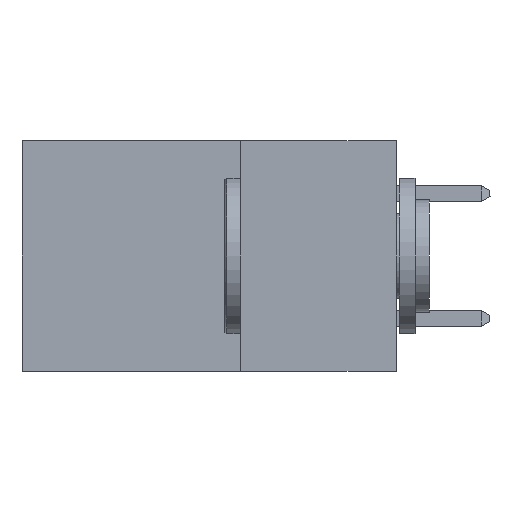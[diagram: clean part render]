
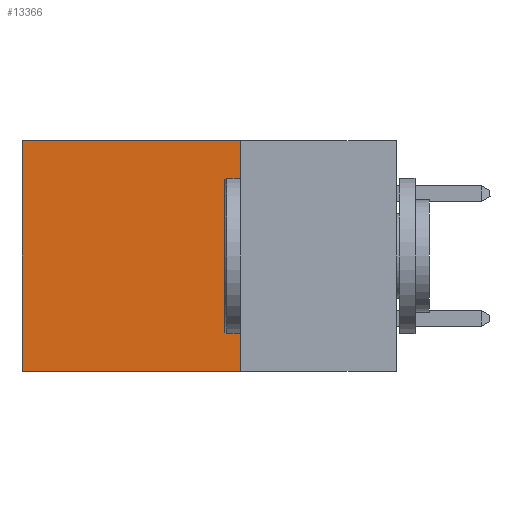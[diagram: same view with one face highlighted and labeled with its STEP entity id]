
A CAD part, left-side view. The second image highlights one B-rep face of the part: STEP entity #13366.
In plain terms, the highlighted planar face has unit normal (-1, 0, 0).
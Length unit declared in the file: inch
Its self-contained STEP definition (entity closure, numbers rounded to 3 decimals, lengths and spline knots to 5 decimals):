
#892 = CARTESIAN_POINT ( 'NONE',  ( 0.298, 0.6, 0. ) ) ;
#2331 = EDGE_CURVE ( 'NONE', #17434, #15738, #8246, .T. ) ;
#3453 = EDGE_CURVE ( 'NONE', #25049, #17434, #6326, .T. ) ;
#4589 = PLANE ( 'NONE',  #15478 ) ;
#4840 = VECTOR ( 'NONE', #21084, 39.37008 ) ;
#6326 = LINE ( 'NONE', #29854, #23415 ) ;
#7138 = DIRECTION ( 'NONE',  ( 0., 1., 0. ) ) ;
#7396 = CARTESIAN_POINT ( 'NONE',  ( 0.298, 0.25, -0.37 ) ) ;
#8246 = LINE ( 'NONE', #11074, #10422 ) ;
#9672 = ORIENTED_EDGE ( 'NONE', *, *, #22484, .T. ) ;
#10234 = ORIENTED_EDGE ( 'NONE', *, *, #16487, .T. ) ;
#10422 = VECTOR ( 'NONE', #7138, 39.37008 ) ;
#11074 = CARTESIAN_POINT ( 'NONE',  ( 0.298, 0.25, -0.37 ) ) ;
#11639 = DIRECTION ( 'NONE',  ( 1., 0., 0. ) ) ;
#12233 = VECTOR ( 'NONE', #15366, 39.37008 ) ;
#12458 = CARTESIAN_POINT ( 'NONE',  ( 0.298, 0.25, 0. ) ) ;
#13366 = ADVANCED_FACE ( 'NONE', ( #21396 ), #4589, .F. ) ;
#13510 = ORIENTED_EDGE ( 'NONE', *, *, #2331, .F. ) ;
#14886 = ORIENTED_EDGE ( 'NONE', *, *, #3453, .F. ) ;
#15366 = DIRECTION ( 'NONE',  ( 0., 0., -1. ) ) ;
#15471 = DIRECTION ( 'NONE',  ( 0., 0., -1. ) ) ;
#15478 = AXIS2_PLACEMENT_3D ( 'NONE', #20868, #11639, #27815 ) ;
#15738 = VERTEX_POINT ( 'NONE', #19323 ) ;
#16260 = EDGE_LOOP ( 'NONE', ( #10234, #13510, #14886, #9672 ) ) ;
#16487 = EDGE_CURVE ( 'NONE', #18747, #15738, #24560, .T. ) ;
#17434 = VERTEX_POINT ( 'NONE', #7396 ) ;
#18747 = VERTEX_POINT ( 'NONE', #892 ) ;
#19323 = CARTESIAN_POINT ( 'NONE',  ( 0.298, 0.6, -0.37 ) ) ;
#20868 = CARTESIAN_POINT ( 'NONE',  ( 0.298, 0.25, 0. ) ) ;
#21084 = DIRECTION ( 'NONE',  ( 0., 1., 0. ) ) ;
#21396 = FACE_OUTER_BOUND ( 'NONE', #16260, .T. ) ;
#22484 = EDGE_CURVE ( 'NONE', #25049, #18747, #23413, .T. ) ;
#23413 = LINE ( 'NONE', #23424, #4840 ) ;
#23415 = VECTOR ( 'NONE', #15471, 39.37008 ) ;
#23424 = CARTESIAN_POINT ( 'NONE',  ( 0.298, 0.25, 0. ) ) ;
#24560 = LINE ( 'NONE', #29162, #12233 ) ;
#25049 = VERTEX_POINT ( 'NONE', #12458 ) ;
#27815 = DIRECTION ( 'NONE',  ( 0., 0., -1. ) ) ;
#29162 = CARTESIAN_POINT ( 'NONE',  ( 0.298, 0.6, 0. ) ) ;
#29854 = CARTESIAN_POINT ( 'NONE',  ( 0.298, 0.25, 0. ) ) ;
